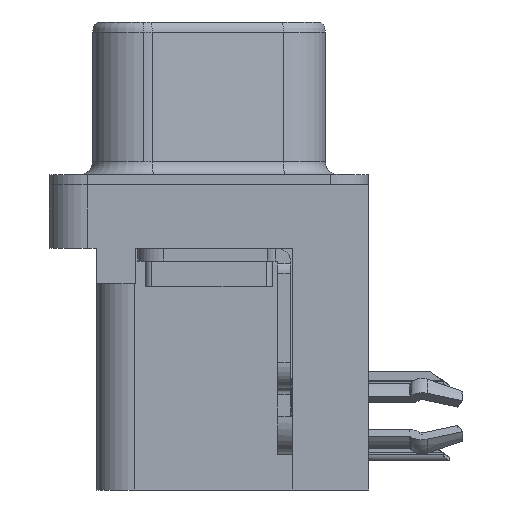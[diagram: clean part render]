
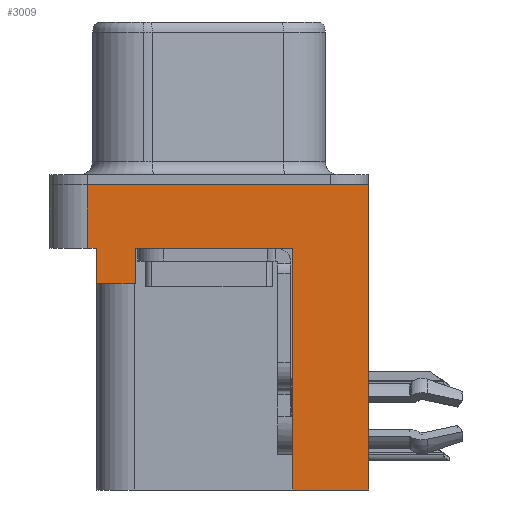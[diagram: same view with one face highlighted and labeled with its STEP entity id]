
A CAD part, left-side view. The second image highlights one B-rep face of the part: STEP entity #3009.
In plain terms, the highlighted planar face has unit normal (-1, 0, 0).
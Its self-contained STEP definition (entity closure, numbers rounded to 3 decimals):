
#136 = ORIENTED_EDGE ( 'NONE', *, *, #21338, .F. ) ;
#324 = VECTOR ( 'NONE', #12304, 1000. ) ;
#454 = EDGE_CURVE ( 'NONE', #15268, #16184, #1466, .T. ) ;
#746 = CARTESIAN_POINT ( 'NONE',  ( -3., 4.425, -3.9 ) ) ;
#757 = CARTESIAN_POINT ( 'NONE',  ( -3., -3.295, -2.5 ) ) ;
#1187 = CARTESIAN_POINT ( 'NONE',  ( -3., -6.275, -2.5 ) ) ;
#1331 = DIRECTION ( 'NONE',  ( 0., 1., 0. ) ) ;
#1466 = LINE ( 'NONE', #19236, #20201 ) ;
#1768 = CARTESIAN_POINT ( 'NONE',  ( -3., 4.775, -2.5 ) ) ;
#2085 = EDGE_CURVE ( 'NONE', #22551, #10173, #22795, .T. ) ;
#2502 = VECTOR ( 'NONE', #11325, 1000. ) ;
#2932 = EDGE_CURVE ( 'NONE', #8999, #22551, #6987, .T. ) ;
#3009 = ADVANCED_FACE ( 'NONE', ( #14727 ), #11169, .T. ) ;
#3645 = EDGE_CURVE ( 'NONE', #18456, #7738, #23004, .T. ) ;
#3933 = EDGE_CURVE ( 'NONE', #21394, #16184, #18250, .T. ) ;
#5126 = DIRECTION ( 'NONE',  ( 0., 0., 1. ) ) ;
#5285 = VECTOR ( 'NONE', #11834, 1000. ) ;
#6006 = LINE ( 'NONE', #6818, #324 ) ;
#6052 = DIRECTION ( 'NONE',  ( 0., 0., 1. ) ) ;
#6309 = ORIENTED_EDGE ( 'NONE', *, *, #7099, .T. ) ;
#6554 = DIRECTION ( 'NONE',  ( 0., 0., 1. ) ) ;
#6818 = CARTESIAN_POINT ( 'NONE',  ( -3., -3.295, -12. ) ) ;
#6987 = LINE ( 'NONE', #13499, #21538 ) ;
#7099 = EDGE_CURVE ( 'NONE', #7853, #7738, #8865, .T. ) ;
#7119 = CARTESIAN_POINT ( 'NONE',  ( -3., -3.295, -12. ) ) ;
#7414 = DIRECTION ( 'NONE',  ( 0., 0., 1. ) ) ;
#7637 = DIRECTION ( 'NONE',  ( 0., 0., 1. ) ) ;
#7738 = VERTEX_POINT ( 'NONE', #13900 ) ;
#7853 = VERTEX_POINT ( 'NONE', #14887 ) ;
#8865 = LINE ( 'NONE', #17947, #22234 ) ;
#8999 = VERTEX_POINT ( 'NONE', #17776 ) ;
#9412 = CARTESIAN_POINT ( 'NONE',  ( -3., -3.295, -12. ) ) ;
#9769 = CARTESIAN_POINT ( 'NONE',  ( -3., -6.275, 0. ) ) ;
#9896 = ORIENTED_EDGE ( 'NONE', *, *, #454, .F. ) ;
#10173 = VERTEX_POINT ( 'NONE', #757 ) ;
#10953 = CARTESIAN_POINT ( 'NONE',  ( -3., 4.425, -3.9 ) ) ;
#11169 = PLANE ( 'NONE',  #19055 ) ;
#11323 = LINE ( 'NONE', #746, #11644 ) ;
#11325 = DIRECTION ( 'NONE',  ( 0., -1., 0. ) ) ;
#11644 = VECTOR ( 'NONE', #17527, 1000. ) ;
#11672 = LINE ( 'NONE', #7119, #19975 ) ;
#11834 = DIRECTION ( 'NONE',  ( 0., -1., 0. ) ) ;
#12304 = DIRECTION ( 'NONE',  ( 0., 0., 1. ) ) ;
#12483 = ORIENTED_EDGE ( 'NONE', *, *, #3645, .F. ) ;
#13205 = ORIENTED_EDGE ( 'NONE', *, *, #3933, .T. ) ;
#13499 = CARTESIAN_POINT ( 'NONE',  ( -3., 2.895, -3.9 ) ) ;
#13900 = CARTESIAN_POINT ( 'NONE',  ( -3., -6.275, 0. ) ) ;
#14727 = FACE_OUTER_BOUND ( 'NONE', #19346, .T. ) ;
#14887 = CARTESIAN_POINT ( 'NONE',  ( -3., -6.275, -12. ) ) ;
#15209 = VECTOR ( 'NONE', #5126, 1000. ) ;
#15268 = VERTEX_POINT ( 'NONE', #10953 ) ;
#15490 = CARTESIAN_POINT ( 'NONE',  ( -3., -6.275, -2.5 ) ) ;
#15561 = CARTESIAN_POINT ( 'NONE',  ( -3., 4.775, 0. ) ) ;
#16184 = VERTEX_POINT ( 'NONE', #20313 ) ;
#16324 = CARTESIAN_POINT ( 'NONE',  ( -3., 4.775, -2.5 ) ) ;
#17006 = VERTEX_POINT ( 'NONE', #9412 ) ;
#17527 = DIRECTION ( 'NONE',  ( 0., 1., 0. ) ) ;
#17776 = CARTESIAN_POINT ( 'NONE',  ( -3., 2.895, -3.9 ) ) ;
#17947 = CARTESIAN_POINT ( 'NONE',  ( -3., -6.275, -2.5 ) ) ;
#18250 = LINE ( 'NONE', #1187, #24244 ) ;
#18456 = VERTEX_POINT ( 'NONE', #15561 ) ;
#18567 = CARTESIAN_POINT ( 'NONE',  ( -3., -6.275, -2.5 ) ) ;
#19055 = AXIS2_PLACEMENT_3D ( 'NONE', #18567, #24537, #7414 ) ;
#19236 = CARTESIAN_POINT ( 'NONE',  ( -3., 4.425, -3.9 ) ) ;
#19346 = EDGE_LOOP ( 'NONE', ( #12483, #136, #13205, #9896, #19897, #22825, #21920, #24596, #21947, #6309 ) ) ;
#19897 = ORIENTED_EDGE ( 'NONE', *, *, #20156, .F. ) ;
#19975 = VECTOR ( 'NONE', #1331, 1000. ) ;
#20156 = EDGE_CURVE ( 'NONE', #8999, #15268, #11323, .T. ) ;
#20191 = EDGE_CURVE ( 'NONE', #17006, #10173, #6006, .T. ) ;
#20201 = VECTOR ( 'NONE', #6052, 1000. ) ;
#20209 = CARTESIAN_POINT ( 'NONE',  ( -3., 2.895, -2.5 ) ) ;
#20283 = DIRECTION ( 'NONE',  ( 0., -1., 0. ) ) ;
#20313 = CARTESIAN_POINT ( 'NONE',  ( -3., 4.425, -2.5 ) ) ;
#21338 = EDGE_CURVE ( 'NONE', #21394, #18456, #21718, .T. ) ;
#21394 = VERTEX_POINT ( 'NONE', #1768 ) ;
#21538 = VECTOR ( 'NONE', #7637, 1000. ) ;
#21718 = LINE ( 'NONE', #16324, #15209 ) ;
#21920 = ORIENTED_EDGE ( 'NONE', *, *, #2085, .T. ) ;
#21947 = ORIENTED_EDGE ( 'NONE', *, *, #23284, .F. ) ;
#22234 = VECTOR ( 'NONE', #6554, 1000. ) ;
#22551 = VERTEX_POINT ( 'NONE', #20209 ) ;
#22795 = LINE ( 'NONE', #15490, #5285 ) ;
#22825 = ORIENTED_EDGE ( 'NONE', *, *, #2932, .T. ) ;
#23004 = LINE ( 'NONE', #9769, #2502 ) ;
#23284 = EDGE_CURVE ( 'NONE', #7853, #17006, #11672, .T. ) ;
#24244 = VECTOR ( 'NONE', #20283, 1000. ) ;
#24537 = DIRECTION ( 'NONE',  ( -1., 0., 0. ) ) ;
#24596 = ORIENTED_EDGE ( 'NONE', *, *, #20191, .F. ) ;
